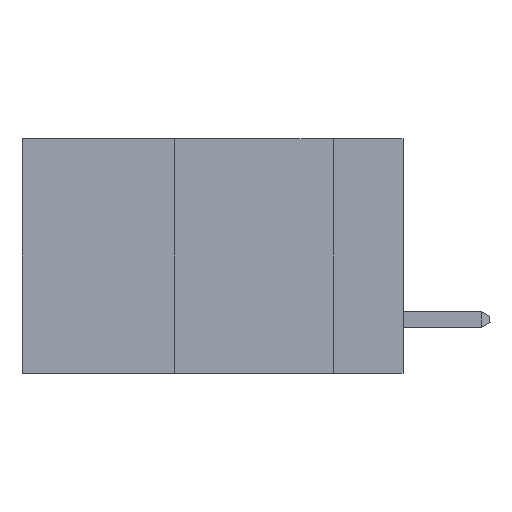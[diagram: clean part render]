
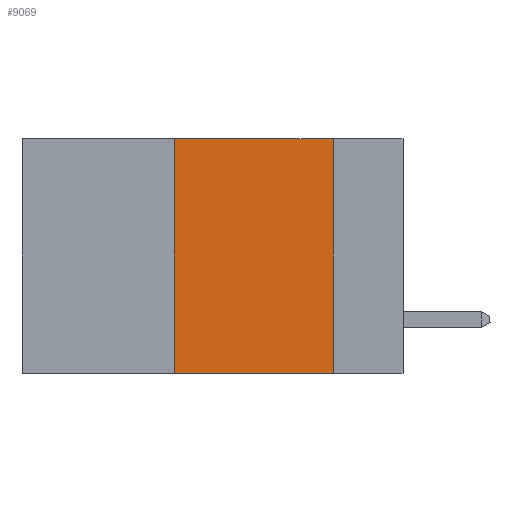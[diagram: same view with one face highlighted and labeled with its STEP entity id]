
A CAD part, left-side view. The second image highlights one B-rep face of the part: STEP entity #9069.
In plain terms, the highlighted planar face has unit normal (-1, 0, 0).
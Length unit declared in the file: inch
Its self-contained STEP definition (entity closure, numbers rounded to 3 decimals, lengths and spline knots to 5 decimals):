
#1135 = LINE ( 'NONE', #28101, #24061 ) ;
#1754 = EDGE_CURVE ( 'NONE', #2511, #33535, #33139, .T. ) ;
#2511 = VERTEX_POINT ( 'NONE', #30388 ) ;
#3990 = CARTESIAN_POINT ( 'NONE',  ( 0., 0.6, 0. ) ) ;
#4951 = LINE ( 'NONE', #34059, #37118 ) ;
#6468 = DIRECTION ( 'NONE',  ( 0., 0., 1. ) ) ;
#7975 = EDGE_CURVE ( 'NONE', #10685, #24147, #17924, .T. ) ;
#9069 = ADVANCED_FACE ( 'NONE', ( #32407 ), #23049, .F. ) ;
#10685 = VERTEX_POINT ( 'NONE', #27922 ) ;
#11389 = DIRECTION ( 'NONE',  ( 0., 0., -1. ) ) ;
#12806 = ORIENTED_EDGE ( 'NONE', *, *, #7975, .T. ) ;
#17924 = LINE ( 'NONE', #28465, #21305 ) ;
#18558 = VECTOR ( 'NONE', #33475, 39.37008 ) ;
#19341 = EDGE_LOOP ( 'NONE', ( #38072, #20764, #34267, #12806 ) ) ;
#20225 = AXIS2_PLACEMENT_3D ( 'NONE', #3990, #29708, #11389 ) ;
#20764 = ORIENTED_EDGE ( 'NONE', *, *, #1754, .F. ) ;
#21305 = VECTOR ( 'NONE', #22600, 39.37008 ) ;
#22600 = DIRECTION ( 'NONE',  ( 0., -1., 0. ) ) ;
#23049 = PLANE ( 'NONE',  #20225 ) ;
#24061 = VECTOR ( 'NONE', #6468, 39.37008 ) ;
#24147 = VERTEX_POINT ( 'NONE', #30397 ) ;
#27922 = CARTESIAN_POINT ( 'NONE',  ( 0., 0.36, -0.37 ) ) ;
#28101 = CARTESIAN_POINT ( 'NONE',  ( 0., 0.36, 0. ) ) ;
#28465 = CARTESIAN_POINT ( 'NONE',  ( 0., 0.6, -0.37 ) ) ;
#29708 = DIRECTION ( 'NONE',  ( 1., 0., 0. ) ) ;
#30388 = CARTESIAN_POINT ( 'NONE',  ( 0., 0.36, 0. ) ) ;
#30397 = CARTESIAN_POINT ( 'NONE',  ( 0., 0.11, -0.37 ) ) ;
#30628 = CARTESIAN_POINT ( 'NONE',  ( 0., 0.11, 0. ) ) ;
#32407 = FACE_OUTER_BOUND ( 'NONE', #19341, .T. ) ;
#33139 = LINE ( 'NONE', #39062, #18558 ) ;
#33475 = DIRECTION ( 'NONE',  ( 0., -1., 0. ) ) ;
#33535 = VERTEX_POINT ( 'NONE', #30628 ) ;
#33708 = EDGE_CURVE ( 'NONE', #33535, #24147, #4951, .T. ) ;
#34059 = CARTESIAN_POINT ( 'NONE',  ( 0., 0.11, 0. ) ) ;
#34267 = ORIENTED_EDGE ( 'NONE', *, *, #37864, .F. ) ;
#37118 = VECTOR ( 'NONE', #40307, 39.37008 ) ;
#37864 = EDGE_CURVE ( 'NONE', #10685, #2511, #1135, .T. ) ;
#38072 = ORIENTED_EDGE ( 'NONE', *, *, #33708, .F. ) ;
#39062 = CARTESIAN_POINT ( 'NONE',  ( 0., 0.6, 0. ) ) ;
#40307 = DIRECTION ( 'NONE',  ( 0., 0., -1. ) ) ;
